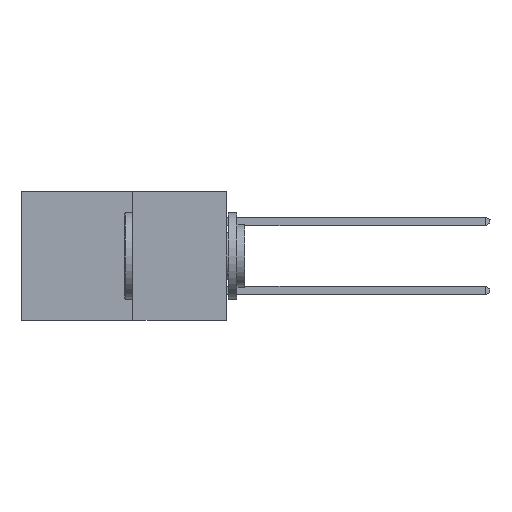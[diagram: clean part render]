
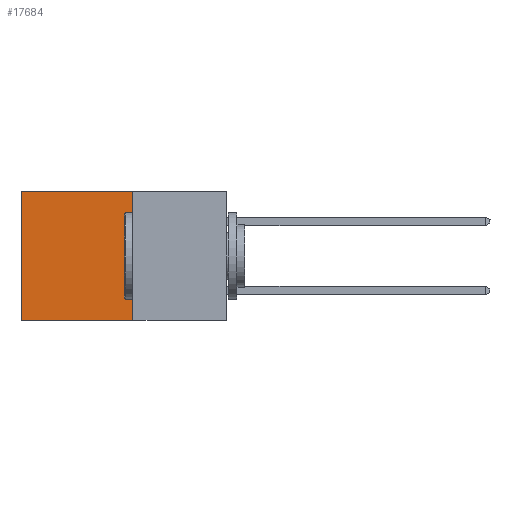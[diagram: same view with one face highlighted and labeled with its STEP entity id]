
A CAD part, left-side view. The second image highlights one B-rep face of the part: STEP entity #17684.
In plain terms, the highlighted planar face has unit normal (-1, 0, 0).
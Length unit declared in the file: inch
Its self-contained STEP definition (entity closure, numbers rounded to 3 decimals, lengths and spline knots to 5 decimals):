
#38 = CARTESIAN_POINT ( 'NONE',  ( 0.277, 0.59, -0.37 ) ) ;
#47 = VECTOR ( 'NONE', #20485, 39.37008 ) ;
#4158 = DIRECTION ( 'NONE',  ( 1., 0., 0. ) ) ;
#4764 = VERTEX_POINT ( 'NONE', #20196 ) ;
#5327 = EDGE_CURVE ( 'NONE', #4764, #6102, #20052, .T. ) ;
#6102 = VERTEX_POINT ( 'NONE', #7657 ) ;
#7179 = VERTEX_POINT ( 'NONE', #14454 ) ;
#7294 = EDGE_LOOP ( 'NONE', ( #7650, #16619, #18217, #14296 ) ) ;
#7392 = PLANE ( 'NONE',  #11275 ) ;
#7650 = ORIENTED_EDGE ( 'NONE', *, *, #11318, .T. ) ;
#7657 = CARTESIAN_POINT ( 'NONE',  ( 0.277, 0.59, 0. ) ) ;
#9165 = LINE ( 'NONE', #19026, #47 ) ;
#9328 = CARTESIAN_POINT ( 'NONE',  ( 0.277, 0.27, -0.37 ) ) ;
#10249 = VECTOR ( 'NONE', #19747, 39.37008 ) ;
#11275 = AXIS2_PLACEMENT_3D ( 'NONE', #13887, #4158, #15483 ) ;
#11318 = EDGE_CURVE ( 'NONE', #6102, #13921, #18729, .T. ) ;
#11669 = VECTOR ( 'NONE', #15067, 39.37008 ) ;
#13238 = EDGE_CURVE ( 'NONE', #4764, #7179, #9165, .T. ) ;
#13887 = CARTESIAN_POINT ( 'NONE',  ( 0.277, 0.27, -0.37 ) ) ;
#13921 = VERTEX_POINT ( 'NONE', #38 ) ;
#14296 = ORIENTED_EDGE ( 'NONE', *, *, #5327, .T. ) ;
#14454 = CARTESIAN_POINT ( 'NONE',  ( 0.277, 0.27, -0.37 ) ) ;
#15067 = DIRECTION ( 'NONE',  ( 0., 1., 0. ) ) ;
#15098 = FACE_OUTER_BOUND ( 'NONE', #7294, .T. ) ;
#15210 = CARTESIAN_POINT ( 'NONE',  ( 0.277, 0.27, 0. ) ) ;
#15483 = DIRECTION ( 'NONE',  ( 0., 0., -1. ) ) ;
#15788 = DIRECTION ( 'NONE',  ( 0., 1., 0. ) ) ;
#15986 = VECTOR ( 'NONE', #15788, 39.37008 ) ;
#16619 = ORIENTED_EDGE ( 'NONE', *, *, #20420, .F. ) ;
#17684 = ADVANCED_FACE ( 'NONE', ( #15098 ), #7392, .F. ) ;
#18217 = ORIENTED_EDGE ( 'NONE', *, *, #13238, .F. ) ;
#18729 = LINE ( 'NONE', #19496, #10249 ) ;
#19026 = CARTESIAN_POINT ( 'NONE',  ( 0.277, 0.27, -0.37 ) ) ;
#19496 = CARTESIAN_POINT ( 'NONE',  ( 0.277, 0.59, -0.37 ) ) ;
#19747 = DIRECTION ( 'NONE',  ( 0., 0., -1. ) ) ;
#20052 = LINE ( 'NONE', #15210, #11669 ) ;
#20115 = LINE ( 'NONE', #9328, #15986 ) ;
#20196 = CARTESIAN_POINT ( 'NONE',  ( 0.277, 0.27, 0. ) ) ;
#20420 = EDGE_CURVE ( 'NONE', #7179, #13921, #20115, .T. ) ;
#20485 = DIRECTION ( 'NONE',  ( 0., 0., -1. ) ) ;
